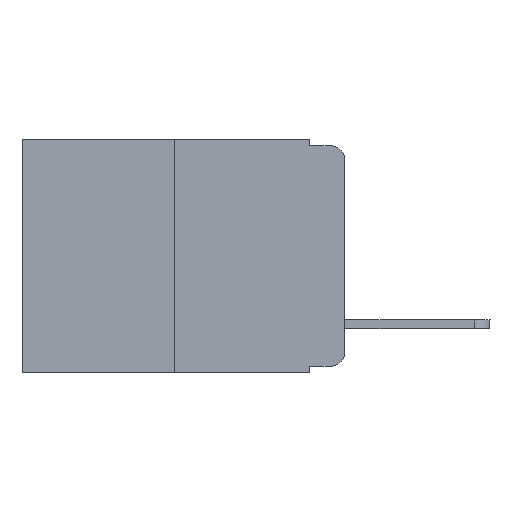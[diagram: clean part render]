
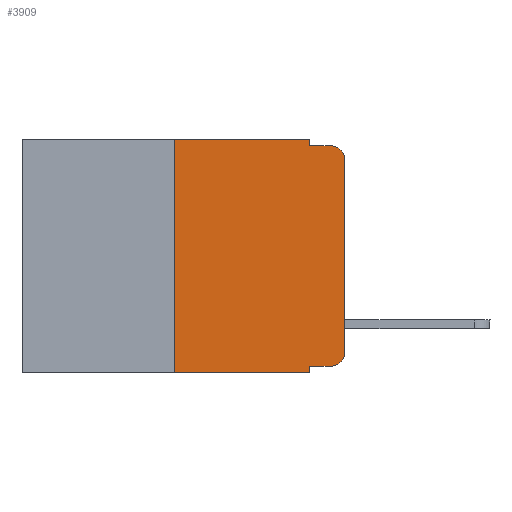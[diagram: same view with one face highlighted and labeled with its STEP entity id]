
A CAD part, left-side view. The second image highlights one B-rep face of the part: STEP entity #3909.
In plain terms, the highlighted planar face has unit normal (-1, 0, 0).
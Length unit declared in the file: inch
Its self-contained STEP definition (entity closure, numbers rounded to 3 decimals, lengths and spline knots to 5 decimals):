
#755 = DIRECTION ( 'NONE',  ( 0., -1., 0. ) ) ;
#1034 = CARTESIAN_POINT ( 'NONE',  ( 0., 0.02, -0.01 ) ) ;
#1036 = ORIENTED_EDGE ( 'NONE', *, *, #17233, .T. ) ;
#1293 = CARTESIAN_POINT ( 'NONE',  ( 0., 0., -0.03 ) ) ;
#1298 = DIRECTION ( 'NONE',  ( 0., 0., -1. ) ) ;
#1343 = LINE ( 'NONE', #8074, #3286 ) ;
#1417 = VERTEX_POINT ( 'NONE', #19100 ) ;
#1937 = DIRECTION ( 'NONE',  ( 0., 0., -1. ) ) ;
#2143 = DIRECTION ( 'NONE',  ( 0., 0., -1. ) ) ;
#2857 = EDGE_CURVE ( 'NONE', #1417, #20782, #19069, .T. ) ;
#3168 = CARTESIAN_POINT ( 'NONE',  ( 0., 0.02, -0.03 ) ) ;
#3286 = VECTOR ( 'NONE', #14790, 39.37008 ) ;
#3897 = CARTESIAN_POINT ( 'NONE',  ( 0., 0.473, -0.343 ) ) ;
#3909 = ADVANCED_FACE ( 'NONE', ( #10205 ), #17043, .F. ) ;
#4428 = ORIENTED_EDGE ( 'NONE', *, *, #6295, .F. ) ;
#4454 = EDGE_LOOP ( 'NONE', ( #7058, #15697, #16293, #17613, #16878, #8273, #14715, #4428, #1036, #20858 ) ) ;
#4500 = EDGE_CURVE ( 'NONE', #4929, #9239, #12397, .T. ) ;
#4540 = VECTOR ( 'NONE', #15786, 39.37008 ) ;
#4730 = EDGE_CURVE ( 'NONE', #18820, #14334, #21456, .T. ) ;
#4929 = VERTEX_POINT ( 'NONE', #5526 ) ;
#5244 = LINE ( 'NONE', #10187, #13673 ) ;
#5376 = CIRCLE ( 'NONE', #17679, 0.02 ) ;
#5478 = DIRECTION ( 'NONE',  ( 0., 0., 1. ) ) ;
#5526 = CARTESIAN_POINT ( 'NONE',  ( 0., 0.25, -0.343 ) ) ;
#5726 = AXIS2_PLACEMENT_3D ( 'NONE', #17479, #20631, #17581 ) ;
#6282 = LINE ( 'NONE', #10006, #14288 ) ;
#6295 = EDGE_CURVE ( 'NONE', #10160, #9239, #6282, .T. ) ;
#6410 = CARTESIAN_POINT ( 'NONE',  ( 0., 0.473, 0. ) ) ;
#6800 = VERTEX_POINT ( 'NONE', #1293 ) ;
#7013 = LINE ( 'NONE', #20527, #8309 ) ;
#7058 = ORIENTED_EDGE ( 'NONE', *, *, #16569, .T. ) ;
#7460 = CARTESIAN_POINT ( 'NONE',  ( 0., 0., 0. ) ) ;
#7911 = CARTESIAN_POINT ( 'NONE',  ( 0., 0.051, -0.01 ) ) ;
#8074 = CARTESIAN_POINT ( 'NONE',  ( 0., 0.051, -0.333 ) ) ;
#8240 = EDGE_CURVE ( 'NONE', #4929, #18820, #7013, .T. ) ;
#8273 = ORIENTED_EDGE ( 'NONE', *, *, #8240, .F. ) ;
#8309 = VECTOR ( 'NONE', #5478, 39.37008 ) ;
#8883 = CARTESIAN_POINT ( 'NONE',  ( 0., 0.25, 0. ) ) ;
#9239 = VERTEX_POINT ( 'NONE', #20113 ) ;
#9261 = VECTOR ( 'NONE', #15715, 39.37008 ) ;
#10006 = CARTESIAN_POINT ( 'NONE',  ( 0., 0.051, 0. ) ) ;
#10160 = VERTEX_POINT ( 'NONE', #15497 ) ;
#10187 = CARTESIAN_POINT ( 'NONE',  ( 0., 0.051, 0. ) ) ;
#10205 = FACE_OUTER_BOUND ( 'NONE', #4454, .T. ) ;
#10235 = CARTESIAN_POINT ( 'NONE',  ( 0., 0.051, -0.01 ) ) ;
#10476 = CARTESIAN_POINT ( 'NONE',  ( 0., 0.051, 0. ) ) ;
#10595 = EDGE_CURVE ( 'NONE', #14334, #16034, #5244, .T. ) ;
#11584 = EDGE_CURVE ( 'NONE', #16034, #17624, #21292, .T. ) ;
#11830 = CARTESIAN_POINT ( 'NONE',  ( 0., 0., -0.313 ) ) ;
#12397 = LINE ( 'NONE', #3897, #4540 ) ;
#13641 = DIRECTION ( 'NONE',  ( 1., 0., 0. ) ) ;
#13673 = VECTOR ( 'NONE', #2143, 39.37008 ) ;
#13965 = CARTESIAN_POINT ( 'NONE',  ( 0., 0.473, 0. ) ) ;
#14288 = VECTOR ( 'NONE', #18373, 39.37008 ) ;
#14334 = VERTEX_POINT ( 'NONE', #10476 ) ;
#14715 = ORIENTED_EDGE ( 'NONE', *, *, #4500, .T. ) ;
#14790 = DIRECTION ( 'NONE',  ( 0., -1., 0. ) ) ;
#15143 = VECTOR ( 'NONE', #19830, 39.37008 ) ;
#15497 = CARTESIAN_POINT ( 'NONE',  ( 0., 0.051, -0.333 ) ) ;
#15697 = ORIENTED_EDGE ( 'NONE', *, *, #16210, .T. ) ;
#15715 = DIRECTION ( 'NONE',  ( 0., 0., 1. ) ) ;
#15786 = DIRECTION ( 'NONE',  ( 0., -1., 0. ) ) ;
#16034 = VERTEX_POINT ( 'NONE', #10235 ) ;
#16210 = EDGE_CURVE ( 'NONE', #6800, #17624, #5376, .T. ) ;
#16293 = ORIENTED_EDGE ( 'NONE', *, *, #11584, .F. ) ;
#16396 = DIRECTION ( 'NONE',  ( -1., 0., 0. ) ) ;
#16569 = EDGE_CURVE ( 'NONE', #20782, #6800, #17261, .T. ) ;
#16847 = AXIS2_PLACEMENT_3D ( 'NONE', #13965, #13641, #1937 ) ;
#16878 = ORIENTED_EDGE ( 'NONE', *, *, #4730, .F. ) ;
#17043 = PLANE ( 'NONE',  #16847 ) ;
#17233 = EDGE_CURVE ( 'NONE', #10160, #1417, #1343, .T. ) ;
#17261 = LINE ( 'NONE', #7460, #9261 ) ;
#17479 = CARTESIAN_POINT ( 'NONE',  ( 0., 0.02, -0.313 ) ) ;
#17581 = DIRECTION ( 'NONE',  ( 0., 0., -1. ) ) ;
#17613 = ORIENTED_EDGE ( 'NONE', *, *, #10595, .F. ) ;
#17624 = VERTEX_POINT ( 'NONE', #1034 ) ;
#17679 = AXIS2_PLACEMENT_3D ( 'NONE', #3168, #16396, #1298 ) ;
#18373 = DIRECTION ( 'NONE',  ( 0., 0., -1. ) ) ;
#18820 = VERTEX_POINT ( 'NONE', #8883 ) ;
#19069 = CIRCLE ( 'NONE', #5726, 0.02 ) ;
#19100 = CARTESIAN_POINT ( 'NONE',  ( 0., 0.02, -0.333 ) ) ;
#19830 = DIRECTION ( 'NONE',  ( 0., -1., 0. ) ) ;
#20113 = CARTESIAN_POINT ( 'NONE',  ( 0., 0.051, -0.343 ) ) ;
#20527 = CARTESIAN_POINT ( 'NONE',  ( 0., 0.25, 0. ) ) ;
#20631 = DIRECTION ( 'NONE',  ( -1., 0., 0. ) ) ;
#20782 = VERTEX_POINT ( 'NONE', #11830 ) ;
#20858 = ORIENTED_EDGE ( 'NONE', *, *, #2857, .T. ) ;
#21292 = LINE ( 'NONE', #7911, #21404 ) ;
#21404 = VECTOR ( 'NONE', #755, 39.37008 ) ;
#21456 = LINE ( 'NONE', #6410, #15143 ) ;
